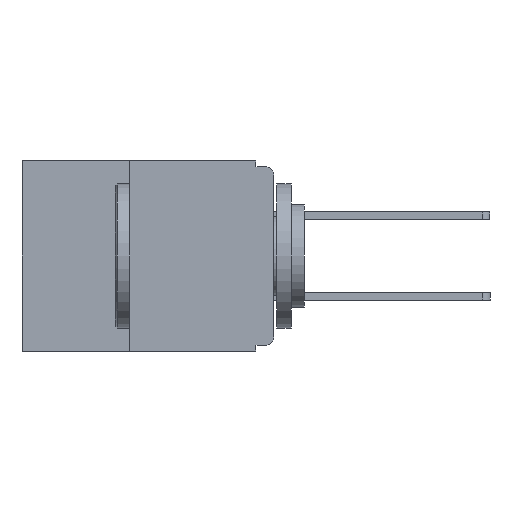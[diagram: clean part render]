
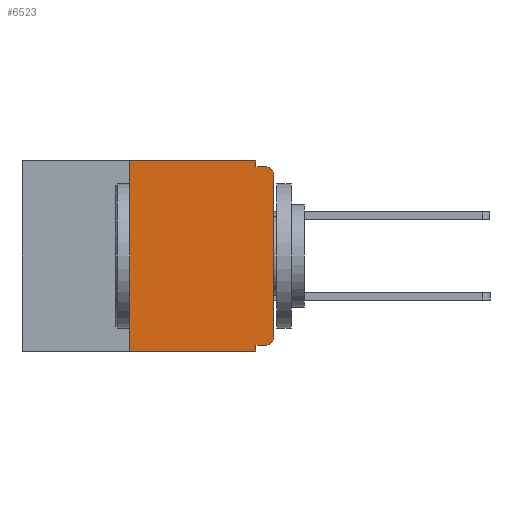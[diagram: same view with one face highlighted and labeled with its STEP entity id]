
A CAD part, left-side view. The second image highlights one B-rep face of the part: STEP entity #6523.
In plain terms, the highlighted planar face has unit normal (-1, 0, 0).
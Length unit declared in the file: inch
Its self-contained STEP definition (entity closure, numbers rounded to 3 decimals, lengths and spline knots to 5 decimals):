
#49 = ORIENTED_EDGE ( 'NONE', *, *, #534, .F. ) ;
#92 = AXIS2_PLACEMENT_3D ( 'NONE', #4246, #16178, #5998 ) ;
#254 = VERTEX_POINT ( 'NONE', #13678 ) ;
#534 = EDGE_CURVE ( 'NONE', #2934, #254, #15241, .T. ) ;
#774 = ORIENTED_EDGE ( 'NONE', *, *, #18769, .T. ) ;
#962 = VECTOR ( 'NONE', #12168, 39.37008 ) ;
#998 = CIRCLE ( 'NONE', #92, 0.015 ) ;
#1122 = CARTESIAN_POINT ( 'NONE',  ( 0., 0.25, -0.33 ) ) ;
#1426 = VECTOR ( 'NONE', #11031, 39.37008 ) ;
#1643 = CARTESIAN_POINT ( 'NONE',  ( 0., 0.015, -0.32 ) ) ;
#1957 = ORIENTED_EDGE ( 'NONE', *, *, #12556, .T. ) ;
#2200 = ORIENTED_EDGE ( 'NONE', *, *, #9097, .T. ) ;
#2789 = LINE ( 'NONE', #16136, #19162 ) ;
#2934 = VERTEX_POINT ( 'NONE', #1643 ) ;
#2944 = ORIENTED_EDGE ( 'NONE', *, *, #8204, .F. ) ;
#3064 = EDGE_CURVE ( 'NONE', #6440, #19288, #6592, .T. ) ;
#3203 = VECTOR ( 'NONE', #11941, 39.37008 ) ;
#3323 = CARTESIAN_POINT ( 'NONE',  ( 0., 0., -0.025 ) ) ;
#3715 = VECTOR ( 'NONE', #11491, 39.37008 ) ;
#4246 = CARTESIAN_POINT ( 'NONE',  ( 0., 0.015, -0.025 ) ) ;
#5304 = FACE_OUTER_BOUND ( 'NONE', #14251, .T. ) ;
#5844 = CARTESIAN_POINT ( 'NONE',  ( 0., 0.437, 0. ) ) ;
#5848 = DIRECTION ( 'NONE',  ( 0., -1., 0. ) ) ;
#5966 = VERTEX_POINT ( 'NONE', #20298 ) ;
#5998 = DIRECTION ( 'NONE',  ( 0., 0., -1. ) ) ;
#6284 = ORIENTED_EDGE ( 'NONE', *, *, #13968, .F. ) ;
#6440 = VERTEX_POINT ( 'NONE', #12652 ) ;
#6523 = ADVANCED_FACE ( 'NONE', ( #5304 ), #11406, .F. ) ;
#6592 = LINE ( 'NONE', #5844, #1426 ) ;
#7335 = CARTESIAN_POINT ( 'NONE',  ( 0., 0., -0.01 ) ) ;
#7834 = CARTESIAN_POINT ( 'NONE',  ( 0., 0.015, -0.305 ) ) ;
#7851 = DIRECTION ( 'NONE',  ( -1., 0., 0. ) ) ;
#7880 = DIRECTION ( 'NONE',  ( 0., 0., -1. ) ) ;
#8002 = LINE ( 'NONE', #8519, #12058 ) ;
#8204 = EDGE_CURVE ( 'NONE', #254, #20492, #2789, .T. ) ;
#8297 = LINE ( 'NONE', #1122, #3715 ) ;
#8519 = CARTESIAN_POINT ( 'NONE',  ( 0., 0.031, 0. ) ) ;
#8639 = VERTEX_POINT ( 'NONE', #3323 ) ;
#8804 = CARTESIAN_POINT ( 'NONE',  ( 0., 0.015, -0.01 ) ) ;
#9097 = EDGE_CURVE ( 'NONE', #2934, #19946, #11919, .T. ) ;
#9469 = CARTESIAN_POINT ( 'NONE',  ( 0., 0.031, -0.33 ) ) ;
#9841 = EDGE_CURVE ( 'NONE', #5966, #21437, #14808, .T. ) ;
#10215 = CARTESIAN_POINT ( 'NONE',  ( 0., 0., 0. ) ) ;
#10259 = VECTOR ( 'NONE', #5848, 39.37008 ) ;
#11031 = DIRECTION ( 'NONE',  ( 0., -1., 0. ) ) ;
#11097 = DIRECTION ( 'NONE',  ( 0., 0., -1. ) ) ;
#11112 = DIRECTION ( 'NONE',  ( 1., 0., 0. ) ) ;
#11406 = PLANE ( 'NONE',  #15346 ) ;
#11491 = DIRECTION ( 'NONE',  ( 0., 0., 1. ) ) ;
#11555 = CARTESIAN_POINT ( 'NONE',  ( 0., 0.437, 0. ) ) ;
#11611 = CARTESIAN_POINT ( 'NONE',  ( 0., 0.031, 0. ) ) ;
#11813 = CARTESIAN_POINT ( 'NONE',  ( 0., 0., -0.305 ) ) ;
#11919 = CIRCLE ( 'NONE', #14288, 0.015 ) ;
#11941 = DIRECTION ( 'NONE',  ( 0., 0., 1. ) ) ;
#12058 = VECTOR ( 'NONE', #16992, 39.37008 ) ;
#12168 = DIRECTION ( 'NONE',  ( 0., 1., 0. ) ) ;
#12556 = EDGE_CURVE ( 'NONE', #8639, #21437, #998, .T. ) ;
#12652 = CARTESIAN_POINT ( 'NONE',  ( 0., 0.25, 0. ) ) ;
#12661 = LINE ( 'NONE', #13568, #17050 ) ;
#12822 = EDGE_CURVE ( 'NONE', #17282, #20492, #12661, .T. ) ;
#13289 = CARTESIAN_POINT ( 'NONE',  ( 0., 0., -0.32 ) ) ;
#13412 = ORIENTED_EDGE ( 'NONE', *, *, #19399, .F. ) ;
#13435 = ORIENTED_EDGE ( 'NONE', *, *, #9841, .F. ) ;
#13568 = CARTESIAN_POINT ( 'NONE',  ( 0., 0.437, -0.33 ) ) ;
#13678 = CARTESIAN_POINT ( 'NONE',  ( 0., 0.031, -0.32 ) ) ;
#13968 = EDGE_CURVE ( 'NONE', #17282, #6440, #8297, .T. ) ;
#14251 = EDGE_LOOP ( 'NONE', ( #774, #1957, #13435, #13412, #18227, #6284, #19286, #2944, #49, #2200 ) ) ;
#14288 = AXIS2_PLACEMENT_3D ( 'NONE', #7834, #7851, #7880 ) ;
#14808 = LINE ( 'NONE', #7335, #10259 ) ;
#15241 = LINE ( 'NONE', #13289, #962 ) ;
#15242 = DIRECTION ( 'NONE',  ( 0., -1., 0. ) ) ;
#15346 = AXIS2_PLACEMENT_3D ( 'NONE', #11555, #11112, #11097 ) ;
#16136 = CARTESIAN_POINT ( 'NONE',  ( 0., 0.031, -0.33 ) ) ;
#16178 = DIRECTION ( 'NONE',  ( -1., 0., 0. ) ) ;
#16252 = DIRECTION ( 'NONE',  ( 0., 0., -1. ) ) ;
#16992 = DIRECTION ( 'NONE',  ( 0., 0., -1. ) ) ;
#17050 = VECTOR ( 'NONE', #15242, 39.37008 ) ;
#17282 = VERTEX_POINT ( 'NONE', #19264 ) ;
#17784 = LINE ( 'NONE', #10215, #3203 ) ;
#18227 = ORIENTED_EDGE ( 'NONE', *, *, #3064, .F. ) ;
#18769 = EDGE_CURVE ( 'NONE', #19946, #8639, #17784, .T. ) ;
#19162 = VECTOR ( 'NONE', #16252, 39.37008 ) ;
#19264 = CARTESIAN_POINT ( 'NONE',  ( 0., 0.25, -0.33 ) ) ;
#19286 = ORIENTED_EDGE ( 'NONE', *, *, #12822, .T. ) ;
#19288 = VERTEX_POINT ( 'NONE', #11611 ) ;
#19399 = EDGE_CURVE ( 'NONE', #19288, #5966, #8002, .T. ) ;
#19946 = VERTEX_POINT ( 'NONE', #11813 ) ;
#20298 = CARTESIAN_POINT ( 'NONE',  ( 0., 0.031, -0.01 ) ) ;
#20492 = VERTEX_POINT ( 'NONE', #9469 ) ;
#21437 = VERTEX_POINT ( 'NONE', #8804 ) ;
